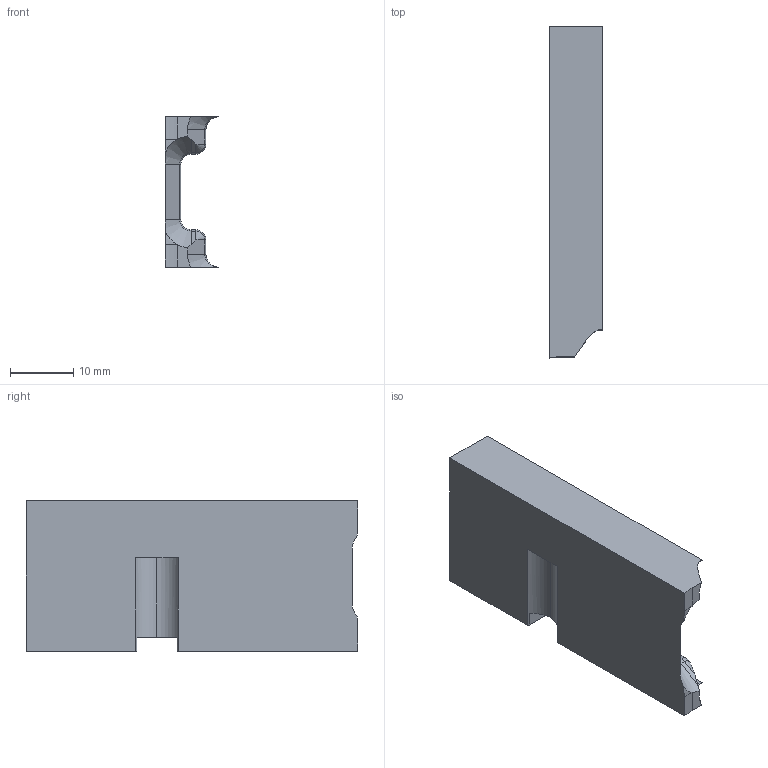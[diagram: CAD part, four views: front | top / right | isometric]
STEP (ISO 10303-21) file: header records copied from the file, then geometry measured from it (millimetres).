
FILE_DESCRIPTION (( 'STEP AP214' ), '1' );
FILE_NAME ('Receiver_Magwell_Rear.step', '2014-05-14T06:10:01', ( 'WarFairy' ), ( '' ), 'SwSTEP 2.0', 'SolidWorks 2013', '' );
FILE_SCHEMA (( 'AUTOMOTIVE_DESIGN' ));
Length unit declared in the file: inch
Products named in the file (1): Receiver_Magwell_Rear
Bounding box: 8.4 x 52.34 x 23.7 mm (x, y, z)
Volume: 5135.8 mm3; surface area: 3841.3 mm2
Topology: 1 solids, 1 shells, 53 faces, 135 edges, 82 vertices
Faces by surface type: plane 23, cylinder 16, cone 6, torus 6, bspline 2
Entity records: 1743 total; most frequent: CARTESIAN_POINT 445, ORIENTED_EDGE 266, DIRECTION 263, EDGE_CURVE 133, AXIS2_PLACEMENT_3D 94, VERTEX_POINT 82, LINE 75, VECTOR 75
